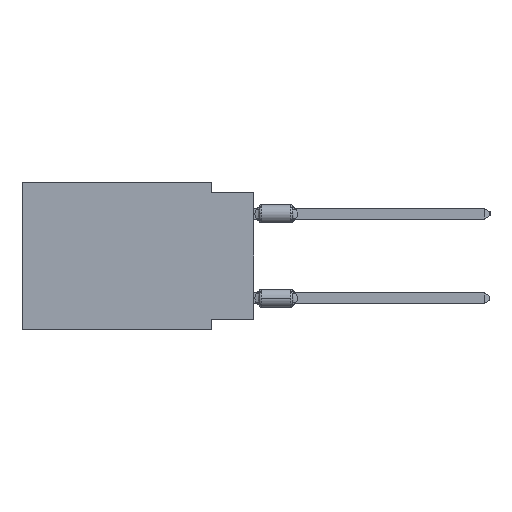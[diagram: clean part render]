
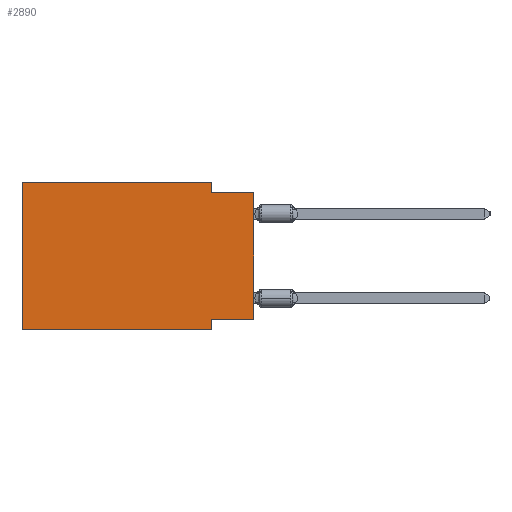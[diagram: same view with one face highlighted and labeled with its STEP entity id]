
A CAD part, left-side view. The second image highlights one B-rep face of the part: STEP entity #2890.
In plain terms, the highlighted planar face has unit normal (-1, 0, 0).
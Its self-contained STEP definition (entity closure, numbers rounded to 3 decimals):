
#159 = ORIENTED_EDGE ( 'NONE', *, *, #30954, .T. ) ;
#2890 = ADVANCED_FACE ( 'NONE', ( #19331 ), #15120, .F. ) ;
#2971 = VECTOR ( 'NONE', #13037, 1000. ) ;
#4054 = CARTESIAN_POINT ( 'NONE',  ( 0., 0., -0.635 ) ) ;
#5076 = CARTESIAN_POINT ( 'NONE',  ( 0., 2.54, -8.89 ) ) ;
#5643 = VERTEX_POINT ( 'NONE', #22376 ) ;
#5753 = VERTEX_POINT ( 'NONE', #4054 ) ;
#8222 = ORIENTED_EDGE ( 'NONE', *, *, #27731, .F. ) ;
#8513 = CARTESIAN_POINT ( 'NONE',  ( 0., 2.54, 0. ) ) ;
#9378 = VECTOR ( 'NONE', #23960, 1000. ) ;
#9512 = LINE ( 'NONE', #28441, #29430 ) ;
#9537 = CARTESIAN_POINT ( 'NONE',  ( 0., 13.97, -8.89 ) ) ;
#10344 = EDGE_LOOP ( 'NONE', ( #159, #25729, #29374, #8222, #12168, #17804, #22681, #17257 ) ) ;
#11568 = DIRECTION ( 'NONE',  ( 0., 1., 0. ) ) ;
#12168 = ORIENTED_EDGE ( 'NONE', *, *, #20466, .F. ) ;
#12272 = LINE ( 'NONE', #26516, #30702 ) ;
#12454 = DIRECTION ( 'NONE',  ( 0., 0., -1. ) ) ;
#13037 = DIRECTION ( 'NONE',  ( 0., 0., 1. ) ) ;
#13118 = CARTESIAN_POINT ( 'NONE',  ( 0., 13.97, 0. ) ) ;
#13473 = AXIS2_PLACEMENT_3D ( 'NONE', #26556, #29212, #12454 ) ;
#13642 = LINE ( 'NONE', #29639, #2971 ) ;
#13900 = CARTESIAN_POINT ( 'NONE',  ( 0., 0., -8.255 ) ) ;
#14050 = DIRECTION ( 'NONE',  ( 0., 0., -1. ) ) ;
#14115 = VERTEX_POINT ( 'NONE', #5076 ) ;
#14691 = VERTEX_POINT ( 'NONE', #24051 ) ;
#15120 = PLANE ( 'NONE',  #13473 ) ;
#15436 = VECTOR ( 'NONE', #28570, 1000. ) ;
#16729 = DIRECTION ( 'NONE',  ( 0., -1., 0. ) ) ;
#17072 = EDGE_CURVE ( 'NONE', #30525, #14115, #9512, .T. ) ;
#17156 = VECTOR ( 'NONE', #11568, 1000. ) ;
#17257 = ORIENTED_EDGE ( 'NONE', *, *, #26815, .F. ) ;
#17519 = EDGE_CURVE ( 'NONE', #17780, #14691, #21205, .T. ) ;
#17780 = VERTEX_POINT ( 'NONE', #8513 ) ;
#17804 = ORIENTED_EDGE ( 'NONE', *, *, #20217, .T. ) ;
#18126 = CARTESIAN_POINT ( 'NONE',  ( 0., 0., -8.255 ) ) ;
#18892 = VERTEX_POINT ( 'NONE', #18126 ) ;
#19010 = CARTESIAN_POINT ( 'NONE',  ( 0., 2.54, 0. ) ) ;
#19331 = FACE_OUTER_BOUND ( 'NONE', #10344, .T. ) ;
#19377 = LINE ( 'NONE', #9537, #19736 ) ;
#19736 = VECTOR ( 'NONE', #16729, 1000. ) ;
#19804 = EDGE_CURVE ( 'NONE', #14691, #5753, #30868, .T. ) ;
#20217 = EDGE_CURVE ( 'NONE', #5643, #14115, #19377, .T. ) ;
#20270 = VERTEX_POINT ( 'NONE', #26444 ) ;
#20466 = EDGE_CURVE ( 'NONE', #5643, #20270, #25300, .T. ) ;
#20864 = CARTESIAN_POINT ( 'NONE',  ( 0., 2.54, -8.255 ) ) ;
#20878 = VECTOR ( 'NONE', #30175, 1000. ) ;
#21205 = LINE ( 'NONE', #19010, #15436 ) ;
#22376 = CARTESIAN_POINT ( 'NONE',  ( 0., 13.97, -8.89 ) ) ;
#22681 = ORIENTED_EDGE ( 'NONE', *, *, #17072, .F. ) ;
#23960 = DIRECTION ( 'NONE',  ( 0., -1., 0. ) ) ;
#24051 = CARTESIAN_POINT ( 'NONE',  ( 0., 2.54, -0.635 ) ) ;
#25300 = LINE ( 'NONE', #13118, #20878 ) ;
#25729 = ORIENTED_EDGE ( 'NONE', *, *, #19804, .F. ) ;
#26444 = CARTESIAN_POINT ( 'NONE',  ( 0., 13.97, 0. ) ) ;
#26516 = CARTESIAN_POINT ( 'NONE',  ( 0., 13.97, 0. ) ) ;
#26556 = CARTESIAN_POINT ( 'NONE',  ( 0., 13.97, 0. ) ) ;
#26815 = EDGE_CURVE ( 'NONE', #18892, #30525, #30350, .T. ) ;
#27731 = EDGE_CURVE ( 'NONE', #20270, #17780, #12272, .T. ) ;
#28441 = CARTESIAN_POINT ( 'NONE',  ( 0., 2.54, -8.89 ) ) ;
#28570 = DIRECTION ( 'NONE',  ( 0., 0., -1. ) ) ;
#29144 = CARTESIAN_POINT ( 'NONE',  ( 0., 0., -0.635 ) ) ;
#29176 = DIRECTION ( 'NONE',  ( 0., -1., 0. ) ) ;
#29212 = DIRECTION ( 'NONE',  ( 1., 0., 0. ) ) ;
#29374 = ORIENTED_EDGE ( 'NONE', *, *, #17519, .F. ) ;
#29430 = VECTOR ( 'NONE', #14050, 1000. ) ;
#29639 = CARTESIAN_POINT ( 'NONE',  ( 0., 0., 0. ) ) ;
#30175 = DIRECTION ( 'NONE',  ( 0., 0., 1. ) ) ;
#30350 = LINE ( 'NONE', #13900, #17156 ) ;
#30525 = VERTEX_POINT ( 'NONE', #20864 ) ;
#30702 = VECTOR ( 'NONE', #29176, 1000. ) ;
#30868 = LINE ( 'NONE', #29144, #9378 ) ;
#30954 = EDGE_CURVE ( 'NONE', #18892, #5753, #13642, .T. ) ;
